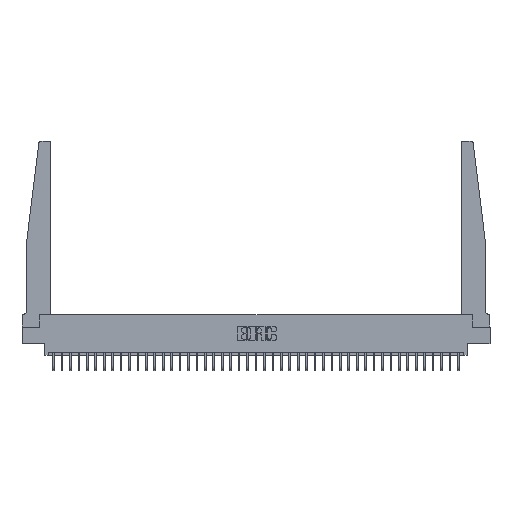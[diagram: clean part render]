
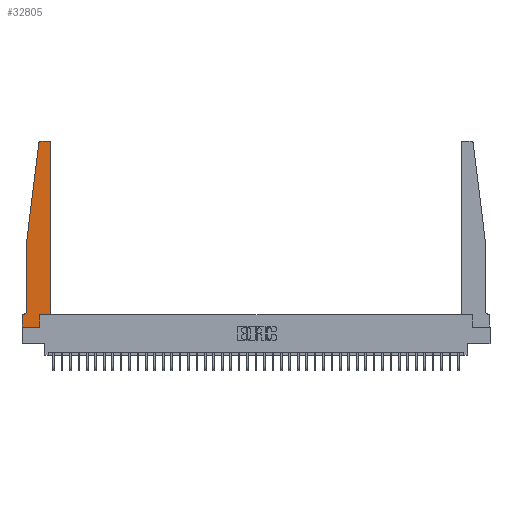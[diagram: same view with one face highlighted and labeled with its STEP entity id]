
A CAD part, top view. The second image highlights one B-rep face of the part: STEP entity #32805.
In plain terms, the highlighted planar face has unit normal (0, 0, 1).
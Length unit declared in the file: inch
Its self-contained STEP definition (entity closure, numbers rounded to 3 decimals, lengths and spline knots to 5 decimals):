
#188 = VERTEX_POINT ( 'NONE', #932 ) ;
#240 = EDGE_CURVE ( 'NONE', #26669, #29003, #305, .T. ) ;
#305 = CIRCLE ( 'NONE', #1379, 0.03 ) ;
#366 = CARTESIAN_POINT ( 'NONE',  ( 0., 0., 0.37 ) ) ;
#595 = LINE ( 'NONE', #20556, #15183 ) ;
#783 = CARTESIAN_POINT ( 'NONE',  ( 0.065, 0.1875, 0.37 ) ) ;
#859 = EDGE_CURVE ( 'NONE', #27472, #20816, #21677, .T. ) ;
#868 = CARTESIAN_POINT ( 'NONE',  ( 0.065, 1.25, 0.37 ) ) ;
#932 = CARTESIAN_POINT ( 'NONE',  ( 0., 0., 0.37 ) ) ;
#1379 = AXIS2_PLACEMENT_3D ( 'NONE', #3956, #4698, #2275 ) ;
#2049 = CIRCLE ( 'NONE', #24670, 0.05 ) ;
#2190 = CIRCLE ( 'NONE', #21109, 0.03 ) ;
#2275 = DIRECTION ( 'NONE',  ( 1., 0., 0. ) ) ;
#2384 = DIRECTION ( 'NONE',  ( 1., 0., 0. ) ) ;
#2873 = ORIENTED_EDGE ( 'NONE', *, *, #4974, .T. ) ;
#3614 = EDGE_CURVE ( 'NONE', #188, #27472, #14033, .T. ) ;
#3659 = VECTOR ( 'NONE', #29099, 39.37008 ) ;
#3956 = CARTESIAN_POINT ( 'NONE',  ( 0.27653, 2.72, 0.37 ) ) ;
#4698 = DIRECTION ( 'NONE',  ( 0., 0., 1. ) ) ;
#4974 = EDGE_CURVE ( 'NONE', #8640, #34079, #29861, .T. ) ;
#5020 = LINE ( 'NONE', #16169, #30047 ) ;
#5022 = ORIENTED_EDGE ( 'NONE', *, *, #20180, .T. ) ;
#5199 = PLANE ( 'NONE',  #12368 ) ;
#5493 = ORIENTED_EDGE ( 'NONE', *, *, #30671, .T. ) ;
#5768 = VERTEX_POINT ( 'NONE', #34712 ) ;
#5951 = DIRECTION ( 'NONE',  ( -1., 0., 0. ) ) ;
#7741 = DIRECTION ( 'NONE',  ( 0., 0., 1. ) ) ;
#8167 = ORIENTED_EDGE ( 'NONE', *, *, #33640, .T. ) ;
#8381 = CARTESIAN_POINT ( 'NONE',  ( 0.25, 2.75, 0.37 ) ) ;
#8460 = ORIENTED_EDGE ( 'NONE', *, *, #33583, .T. ) ;
#8640 = VERTEX_POINT ( 'NONE', #20850 ) ;
#8681 = ORIENTED_EDGE ( 'NONE', *, *, #26567, .T. ) ;
#9140 = VERTEX_POINT ( 'NONE', #36325 ) ;
#9421 = VECTOR ( 'NONE', #16133, 39.37008 ) ;
#10726 = ORIENTED_EDGE ( 'NONE', *, *, #36743, .T. ) ;
#11133 = VERTEX_POINT ( 'NONE', #24568 ) ;
#12368 = AXIS2_PLACEMENT_3D ( 'NONE', #14010, #16894, #2384 ) ;
#12661 = CARTESIAN_POINT ( 'NONE',  ( 0.2605, 0., 0.37 ) ) ;
#14010 = CARTESIAN_POINT ( 'NONE',  ( 0., 0.1875, 0.37 ) ) ;
#14033 = LINE ( 'NONE', #366, #9421 ) ;
#15025 = DIRECTION ( 'NONE',  ( -0.122, -0.992, 0. ) ) ;
#15183 = VECTOR ( 'NONE', #26406, 39.37008 ) ;
#15555 = VECTOR ( 'NONE', #34677, 39.37008 ) ;
#16014 = DIRECTION ( 'NONE',  ( 0., 1., 0. ) ) ;
#16133 = DIRECTION ( 'NONE',  ( 1., 0., 0. ) ) ;
#16169 = CARTESIAN_POINT ( 'NONE',  ( 0.425, 0.18, 0.37 ) ) ;
#16643 = ORIENTED_EDGE ( 'NONE', *, *, #3614, .T. ) ;
#16709 = LINE ( 'NONE', #868, #23490 ) ;
#16894 = DIRECTION ( 'NONE',  ( 0., 0., 1. ) ) ;
#17117 = DIRECTION ( 'NONE',  ( -1., 0., 0. ) ) ;
#17150 = CARTESIAN_POINT ( 'NONE',  ( 0.2605, 0.18, 0.37 ) ) ;
#17342 = EDGE_CURVE ( 'NONE', #9140, #25144, #595, .T. ) ;
#17404 = CARTESIAN_POINT ( 'NONE',  ( 0.24675, 2.72367, 0.37 ) ) ;
#18941 = VECTOR ( 'NONE', #16014, 39.37008 ) ;
#19235 = LINE ( 'NONE', #33083, #21049 ) ;
#19276 = FACE_OUTER_BOUND ( 'NONE', #19621, .T. ) ;
#19621 = EDGE_LOOP ( 'NONE', ( #8167, #27751, #5493, #8460, #8681, #2873, #23586, #16643, #32850, #10726, #31464, #5022 ) ) ;
#20180 = EDGE_CURVE ( 'NONE', #25144, #25577, #2190, .T. ) ;
#20429 = CARTESIAN_POINT ( 'NONE',  ( 0.27653, 2.75, 0.37 ) ) ;
#20556 = CARTESIAN_POINT ( 'NONE',  ( 0.425, 0.18, 0.37 ) ) ;
#20816 = VERTEX_POINT ( 'NONE', #17150 ) ;
#20850 = CARTESIAN_POINT ( 'NONE',  ( 0.015, 0.1875, 0.37 ) ) ;
#21049 = VECTOR ( 'NONE', #21247, 39.37008 ) ;
#21109 = AXIS2_PLACEMENT_3D ( 'NONE', #25181, #7741, #28524 ) ;
#21247 = DIRECTION ( 'NONE',  ( 0., -1., 0. ) ) ;
#21315 = CARTESIAN_POINT ( 'NONE',  ( 0., 0.1875, 0.37 ) ) ;
#21677 = LINE ( 'NONE', #30776, #18941 ) ;
#22413 = LINE ( 'NONE', #8381, #15555 ) ;
#23490 = VECTOR ( 'NONE', #15025, 39.37008 ) ;
#23586 = ORIENTED_EDGE ( 'NONE', *, *, #36257, .T. ) ;
#24568 = CARTESIAN_POINT ( 'NONE',  ( 0.065, 0.2375, 0.37 ) ) ;
#24670 = AXIS2_PLACEMENT_3D ( 'NONE', #37680, #29103, #17117 ) ;
#25144 = VERTEX_POINT ( 'NONE', #26252 ) ;
#25181 = CARTESIAN_POINT ( 'NONE',  ( 0.395, 2.72, 0.37 ) ) ;
#25577 = VERTEX_POINT ( 'NONE', #28578 ) ;
#26252 = CARTESIAN_POINT ( 'NONE',  ( 0.425, 2.72, 0.37 ) ) ;
#26406 = DIRECTION ( 'NONE',  ( 0., 1., 0. ) ) ;
#26567 = EDGE_CURVE ( 'NONE', #11133, #8640, #2049, .T. ) ;
#26669 = VERTEX_POINT ( 'NONE', #20429 ) ;
#27472 = VERTEX_POINT ( 'NONE', #12661 ) ;
#27751 = ORIENTED_EDGE ( 'NONE', *, *, #240, .T. ) ;
#28036 = DIRECTION ( 'NONE',  ( 1., 0., 0. ) ) ;
#28524 = DIRECTION ( 'NONE',  ( 1., 0., 0. ) ) ;
#28578 = CARTESIAN_POINT ( 'NONE',  ( 0.395, 2.75, 0.37 ) ) ;
#29003 = VERTEX_POINT ( 'NONE', #17404 ) ;
#29099 = DIRECTION ( 'NONE',  ( 0., -1., 0. ) ) ;
#29103 = DIRECTION ( 'NONE',  ( 0., 0., -1. ) ) ;
#29861 = LINE ( 'NONE', #783, #35397 ) ;
#30047 = VECTOR ( 'NONE', #28036, 39.37008 ) ;
#30671 = EDGE_CURVE ( 'NONE', #29003, #5768, #16709, .T. ) ;
#30776 = CARTESIAN_POINT ( 'NONE',  ( 0.2605, 0.18, 0.37 ) ) ;
#31464 = ORIENTED_EDGE ( 'NONE', *, *, #17342, .T. ) ;
#32805 = ADVANCED_FACE ( 'NONE', ( #19276 ), #5199, .T. ) ;
#32850 = ORIENTED_EDGE ( 'NONE', *, *, #859, .T. ) ;
#33083 = CARTESIAN_POINT ( 'NONE',  ( 0.065, 1.25, 0.37 ) ) ;
#33583 = EDGE_CURVE ( 'NONE', #5768, #11133, #19235, .T. ) ;
#33640 = EDGE_CURVE ( 'NONE', #25577, #26669, #22413, .T. ) ;
#34079 = VERTEX_POINT ( 'NONE', #21315 ) ;
#34469 = CARTESIAN_POINT ( 'NONE',  ( 0., 0., 0.37 ) ) ;
#34677 = DIRECTION ( 'NONE',  ( -1., 0., 0. ) ) ;
#34712 = CARTESIAN_POINT ( 'NONE',  ( 0.065, 1.25, 0.37 ) ) ;
#35397 = VECTOR ( 'NONE', #5951, 39.37008 ) ;
#36069 = LINE ( 'NONE', #34469, #3659 ) ;
#36257 = EDGE_CURVE ( 'NONE', #34079, #188, #36069, .T. ) ;
#36325 = CARTESIAN_POINT ( 'NONE',  ( 0.425, 0.18, 0.37 ) ) ;
#36743 = EDGE_CURVE ( 'NONE', #20816, #9140, #5020, .T. ) ;
#37680 = CARTESIAN_POINT ( 'NONE',  ( 0.015, 0.2375, 0.37 ) ) ;
